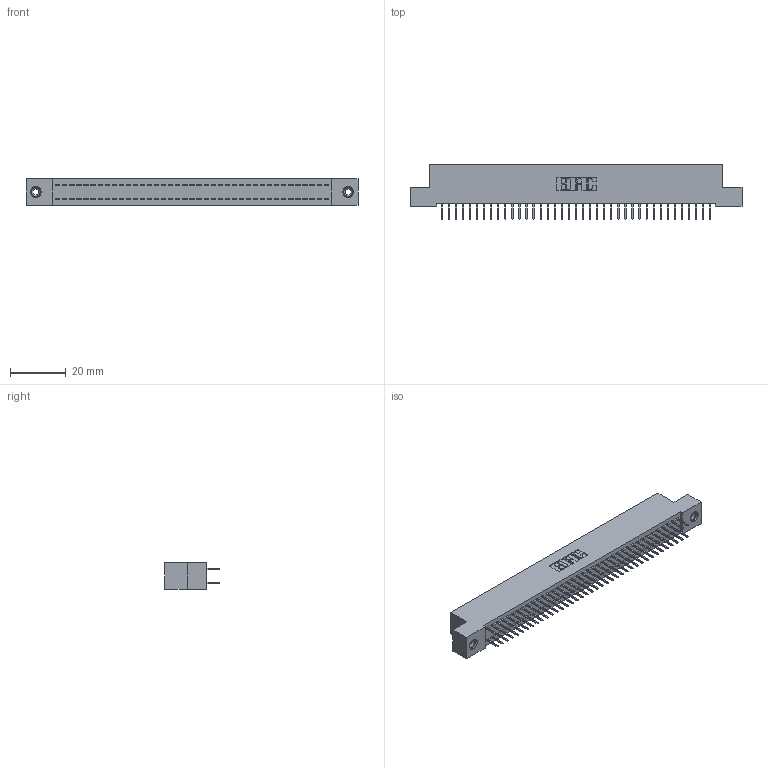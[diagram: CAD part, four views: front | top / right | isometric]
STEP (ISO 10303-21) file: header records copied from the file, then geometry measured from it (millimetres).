
FILE_DESCRIPTION (( 'STEP AP203' ), '1' );
FILE_NAME ('342-078-524-208.STEP', '2019-10-04T11:08:39', ( '' ), ( '' ), 'SwSTEP 2.0', 'SolidWorks 2016', '' );
FILE_SCHEMA (( 'CONFIG_CONTROL_DESIGN' ));
Length unit declared in the file: inch
Products named in the file (4): 342 Part_TI; 345-292-001_345-293-124; 345-250-001_345-250-003-102; 342-078-524-208
Assembly tree (81 placements, depth 2):
  342-078-524-208
    342 Part_TI
    345-292-001_345-293-124  x78
    345-250-001_345-250-003-102  x2
Bounding box: 119.38 x 19.69 x 9.4 mm (x, y, z)
Volume: 10588.4 mm3; surface area: 16864.5 mm2
Topology: 81 solids, 81 shells, 4538 faces, 12837 edges, 8238 vertices
Faces by surface type: plane 3374, cylinder 1148, cone 12, torus 4
Entity records: 26606 total; most frequent: CARTESIAN_POINT 4393, ORIENTED_EDGE 4322, DIRECTION 3791, EDGE_CURVE 2161, VECTOR 2017, LINE 2017, VERTEX_POINT 1432, AXIS2_PLACEMENT_3D 887
